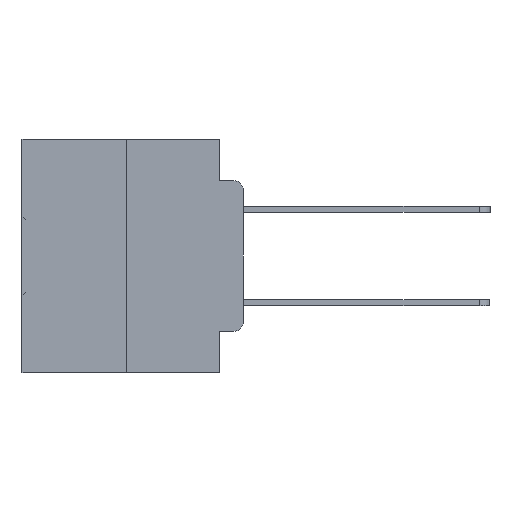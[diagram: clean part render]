
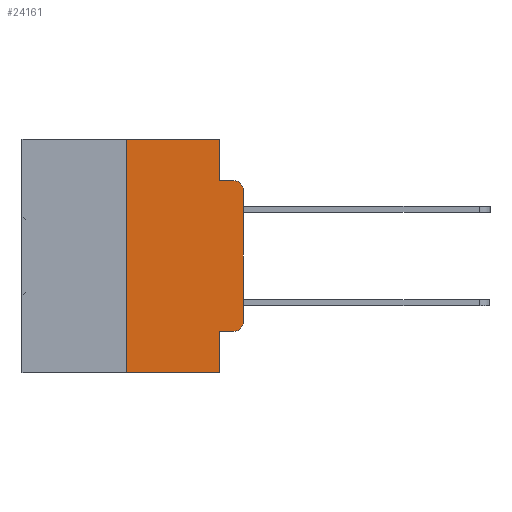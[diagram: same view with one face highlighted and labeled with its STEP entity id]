
A CAD part, left-side view. The second image highlights one B-rep face of the part: STEP entity #24161.
In plain terms, the highlighted planar face has unit normal (-1, 0, 0).
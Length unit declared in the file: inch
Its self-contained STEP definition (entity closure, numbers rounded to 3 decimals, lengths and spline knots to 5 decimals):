
#221 = ORIENTED_EDGE ( 'NONE', *, *, #3182, .T. ) ;
#1115 = CARTESIAN_POINT ( 'NONE',  ( 0., 0.051, -0.0885 ) ) ;
#1467 = ORIENTED_EDGE ( 'NONE', *, *, #19358, .T. ) ;
#1711 = VERTEX_POINT ( 'NONE', #8264 ) ;
#2000 = LINE ( 'NONE', #15870, #29092 ) ;
#2633 = DIRECTION ( 'NONE',  ( 1., 0., 0. ) ) ;
#2680 = DIRECTION ( 'NONE',  ( 0., -1., 0. ) ) ;
#3182 = EDGE_CURVE ( 'NONE', #1711, #4502, #28417, .T. ) ;
#3220 = LINE ( 'NONE', #11350, #30249 ) ;
#3639 = DIRECTION ( 'NONE',  ( 0., -1., 0. ) ) ;
#3807 = DIRECTION ( 'NONE',  ( 0., -1., 0. ) ) ;
#4502 = VERTEX_POINT ( 'NONE', #10141 ) ;
#4667 = CARTESIAN_POINT ( 'NONE',  ( 0., 0.02, -0.0885 ) ) ;
#5342 = VERTEX_POINT ( 'NONE', #14100 ) ;
#5681 = ORIENTED_EDGE ( 'NONE', *, *, #27833, .F. ) ;
#5735 = LINE ( 'NONE', #15751, #25045 ) ;
#5892 = VERTEX_POINT ( 'NONE', #17085 ) ;
#7263 = CIRCLE ( 'NONE', #9099, 0.02 ) ;
#7681 = AXIS2_PLACEMENT_3D ( 'NONE', #18497, #2633, #21137 ) ;
#7858 = DIRECTION ( 'NONE',  ( 0., 0., 1. ) ) ;
#8264 = CARTESIAN_POINT ( 'NONE',  ( 0., 0.051, -0.4115 ) ) ;
#8565 = ORIENTED_EDGE ( 'NONE', *, *, #27197, .F. ) ;
#8854 = VECTOR ( 'NONE', #20655, 39.37008 ) ;
#9099 = AXIS2_PLACEMENT_3D ( 'NONE', #26632, #10990, #29200 ) ;
#9230 = CARTESIAN_POINT ( 'NONE',  ( 0., 0.02, -0.3915 ) ) ;
#9485 = CARTESIAN_POINT ( 'NONE',  ( 0., 0.473, -0.5 ) ) ;
#9824 = EDGE_CURVE ( 'NONE', #5342, #25966, #2000, .T. ) ;
#10141 = CARTESIAN_POINT ( 'NONE',  ( 0., 0.02, -0.4115 ) ) ;
#10230 = CARTESIAN_POINT ( 'NONE',  ( 0., 0.051, 0. ) ) ;
#10495 = LINE ( 'NONE', #25842, #8854 ) ;
#10555 = CARTESIAN_POINT ( 'NONE',  ( 0., 0., -0.3915 ) ) ;
#10645 = AXIS2_PLACEMENT_3D ( 'NONE', #9230, #27496, #11856 ) ;
#10990 = DIRECTION ( 'NONE',  ( -1., 0., 0. ) ) ;
#11350 = CARTESIAN_POINT ( 'NONE',  ( 0., 0.051, 0. ) ) ;
#11856 = DIRECTION ( 'NONE',  ( 0., 0., -1. ) ) ;
#11891 = VERTEX_POINT ( 'NONE', #14184 ) ;
#12109 = DIRECTION ( 'NONE',  ( 0., -1., 0. ) ) ;
#12234 = CARTESIAN_POINT ( 'NONE',  ( 0., 0.25, 0. ) ) ;
#12269 = ORIENTED_EDGE ( 'NONE', *, *, #32934, .F. ) ;
#13111 = VERTEX_POINT ( 'NONE', #4667 ) ;
#13838 = EDGE_CURVE ( 'NONE', #1711, #11891, #10495, .T. ) ;
#14100 = CARTESIAN_POINT ( 'NONE',  ( 0., 0.25, 0. ) ) ;
#14184 = CARTESIAN_POINT ( 'NONE',  ( 0., 0.051, -0.5 ) ) ;
#14296 = EDGE_CURVE ( 'NONE', #5892, #11891, #15756, .T. ) ;
#14942 = VECTOR ( 'NONE', #12109, 39.37008 ) ;
#15751 = CARTESIAN_POINT ( 'NONE',  ( 0., 0., 0. ) ) ;
#15756 = LINE ( 'NONE', #9485, #14942 ) ;
#15870 = CARTESIAN_POINT ( 'NONE',  ( 0., 0.473, 0. ) ) ;
#16022 = CARTESIAN_POINT ( 'NONE',  ( 0., 0.051, -0.0885 ) ) ;
#16303 = VECTOR ( 'NONE', #3807, 39.37008 ) ;
#16771 = ORIENTED_EDGE ( 'NONE', *, *, #14296, .T. ) ;
#17085 = CARTESIAN_POINT ( 'NONE',  ( 0., 0.25, -0.5 ) ) ;
#17205 = ORIENTED_EDGE ( 'NONE', *, *, #9824, .F. ) ;
#17480 = CIRCLE ( 'NONE', #10645, 0.02 ) ;
#18009 = EDGE_LOOP ( 'NONE', ( #18523, #26154, #8565, #12269, #17205, #5681, #16771, #26576, #221, #1467 ) ) ;
#18497 = CARTESIAN_POINT ( 'NONE',  ( 0., 0.473, 0. ) ) ;
#18503 = EDGE_CURVE ( 'NONE', #28927, #13111, #7263, .T. ) ;
#18523 = ORIENTED_EDGE ( 'NONE', *, *, #33363, .T. ) ;
#18810 = VECTOR ( 'NONE', #27846, 39.37008 ) ;
#19358 = EDGE_CURVE ( 'NONE', #4502, #26899, #17480, .T. ) ;
#19529 = CARTESIAN_POINT ( 'NONE',  ( 0., 0., -0.1085 ) ) ;
#20131 = CARTESIAN_POINT ( 'NONE',  ( 0., 0.051, -0.4115 ) ) ;
#20655 = DIRECTION ( 'NONE',  ( 0., 0., -1. ) ) ;
#21137 = DIRECTION ( 'NONE',  ( 0., 0., -1. ) ) ;
#24161 = ADVANCED_FACE ( 'NONE', ( #33108 ), #31356, .F. ) ;
#24949 = LINE ( 'NONE', #12234, #18810 ) ;
#25045 = VECTOR ( 'NONE', #7858, 39.37008 ) ;
#25842 = CARTESIAN_POINT ( 'NONE',  ( 0., 0.051, 0. ) ) ;
#25966 = VERTEX_POINT ( 'NONE', #10230 ) ;
#26154 = ORIENTED_EDGE ( 'NONE', *, *, #18503, .T. ) ;
#26576 = ORIENTED_EDGE ( 'NONE', *, *, #13838, .F. ) ;
#26632 = CARTESIAN_POINT ( 'NONE',  ( 0., 0.02, -0.1085 ) ) ;
#26830 = VECTOR ( 'NONE', #3639, 39.37008 ) ;
#26899 = VERTEX_POINT ( 'NONE', #10555 ) ;
#26949 = VERTEX_POINT ( 'NONE', #16022 ) ;
#27197 = EDGE_CURVE ( 'NONE', #26949, #13111, #30911, .T. ) ;
#27496 = DIRECTION ( 'NONE',  ( -1., 0., 0. ) ) ;
#27833 = EDGE_CURVE ( 'NONE', #5892, #5342, #24949, .T. ) ;
#27846 = DIRECTION ( 'NONE',  ( 0., 0., 1. ) ) ;
#28417 = LINE ( 'NONE', #20131, #26830 ) ;
#28927 = VERTEX_POINT ( 'NONE', #19529 ) ;
#29092 = VECTOR ( 'NONE', #2680, 39.37008 ) ;
#29200 = DIRECTION ( 'NONE',  ( 0., 0., -1. ) ) ;
#29545 = DIRECTION ( 'NONE',  ( 0., 0., -1. ) ) ;
#30249 = VECTOR ( 'NONE', #29545, 39.37008 ) ;
#30911 = LINE ( 'NONE', #1115, #16303 ) ;
#31356 = PLANE ( 'NONE',  #7681 ) ;
#32934 = EDGE_CURVE ( 'NONE', #25966, #26949, #3220, .T. ) ;
#33108 = FACE_OUTER_BOUND ( 'NONE', #18009, .T. ) ;
#33363 = EDGE_CURVE ( 'NONE', #26899, #28927, #5735, .T. ) ;
